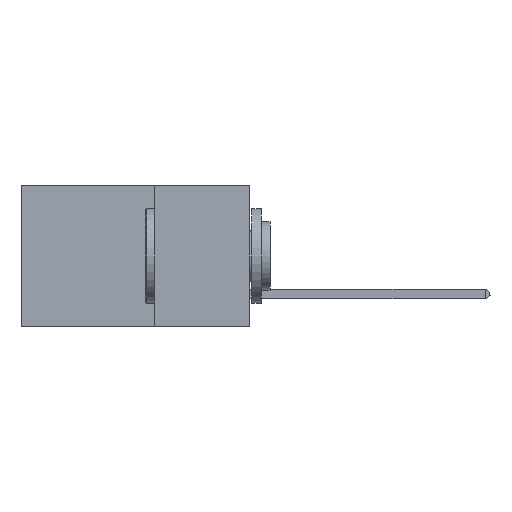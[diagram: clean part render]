
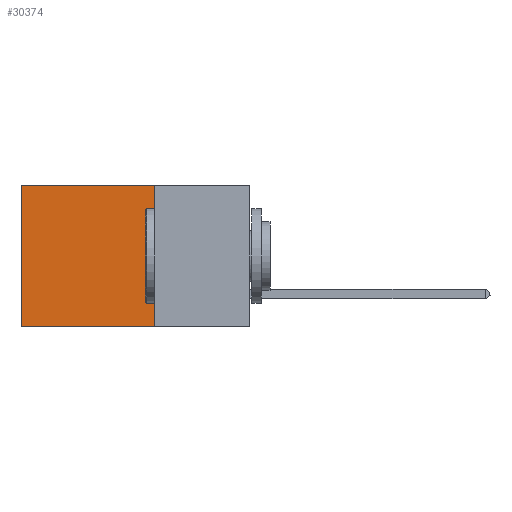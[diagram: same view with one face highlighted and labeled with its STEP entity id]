
A CAD part, left-side view. The second image highlights one B-rep face of the part: STEP entity #30374.
In plain terms, the highlighted planar face has unit normal (-1, 0, 0).
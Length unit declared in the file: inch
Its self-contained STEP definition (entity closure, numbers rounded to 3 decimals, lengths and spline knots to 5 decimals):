
#969 = ORIENTED_EDGE ( 'NONE', *, *, #15897, .F. ) ;
#2833 = VERTEX_POINT ( 'NONE', #37288 ) ;
#8458 = LINE ( 'NONE', #43463, #36636 ) ;
#9097 = VECTOR ( 'NONE', #39598, 39.37008 ) ;
#9898 = DIRECTION ( 'NONE',  ( 1., 0., 0. ) ) ;
#10370 = VERTEX_POINT ( 'NONE', #21875 ) ;
#11180 = FACE_OUTER_BOUND ( 'NONE', #14564, .T. ) ;
#12023 = DIRECTION ( 'NONE',  ( 0., 0., -1. ) ) ;
#14546 = VECTOR ( 'NONE', #43479, 39.37008 ) ;
#14564 = EDGE_LOOP ( 'NONE', ( #38979, #969, #23463, #39197 ) ) ;
#15593 = CARTESIAN_POINT ( 'NONE',  ( 0.2875, 0.25, 0. ) ) ;
#15897 = EDGE_CURVE ( 'NONE', #25352, #38178, #38323, .T. ) ;
#20290 = PLANE ( 'NONE',  #37963 ) ;
#21875 = CARTESIAN_POINT ( 'NONE',  ( 0.2875, 0.6, 0. ) ) ;
#23463 = ORIENTED_EDGE ( 'NONE', *, *, #46752, .F. ) ;
#25352 = VERTEX_POINT ( 'NONE', #46646 ) ;
#26249 = EDGE_CURVE ( 'NONE', #2833, #10370, #37931, .T. ) ;
#26831 = VECTOR ( 'NONE', #12023, 39.37008 ) ;
#28734 = CARTESIAN_POINT ( 'NONE',  ( 0.2875, 0.25, 0. ) ) ;
#30374 = ADVANCED_FACE ( 'NONE', ( #11180 ), #20290, .F. ) ;
#31790 = CARTESIAN_POINT ( 'NONE',  ( 0.2875, 0.25, 0. ) ) ;
#33540 = CARTESIAN_POINT ( 'NONE',  ( 0.2875, 0.6, -0.37 ) ) ;
#35082 = LINE ( 'NONE', #15593, #26831 ) ;
#36636 = VECTOR ( 'NONE', #40841, 39.37008 ) ;
#37288 = CARTESIAN_POINT ( 'NONE',  ( 0.2875, 0.25, 0. ) ) ;
#37931 = LINE ( 'NONE', #28734, #14546 ) ;
#37963 = AXIS2_PLACEMENT_3D ( 'NONE', #31790, #9898, #47542 ) ;
#38178 = VERTEX_POINT ( 'NONE', #33540 ) ;
#38323 = LINE ( 'NONE', #43136, #9097 ) ;
#38979 = ORIENTED_EDGE ( 'NONE', *, *, #40883, .T. ) ;
#39197 = ORIENTED_EDGE ( 'NONE', *, *, #26249, .T. ) ;
#39598 = DIRECTION ( 'NONE',  ( 0., 1., 0. ) ) ;
#40841 = DIRECTION ( 'NONE',  ( 0., 0., -1. ) ) ;
#40883 = EDGE_CURVE ( 'NONE', #10370, #38178, #8458, .T. ) ;
#43136 = CARTESIAN_POINT ( 'NONE',  ( 0.2875, 0.25, -0.37 ) ) ;
#43463 = CARTESIAN_POINT ( 'NONE',  ( 0.2875, 0.6, 0. ) ) ;
#43479 = DIRECTION ( 'NONE',  ( 0., 1., 0. ) ) ;
#46646 = CARTESIAN_POINT ( 'NONE',  ( 0.2875, 0.25, -0.37 ) ) ;
#46752 = EDGE_CURVE ( 'NONE', #2833, #25352, #35082, .T. ) ;
#47542 = DIRECTION ( 'NONE',  ( 0., 0., -1. ) ) ;
